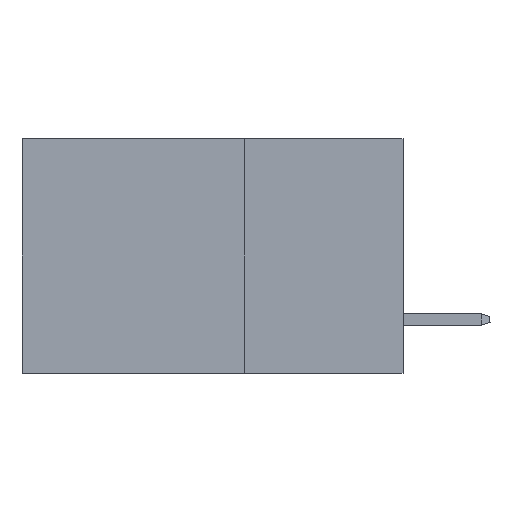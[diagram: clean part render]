
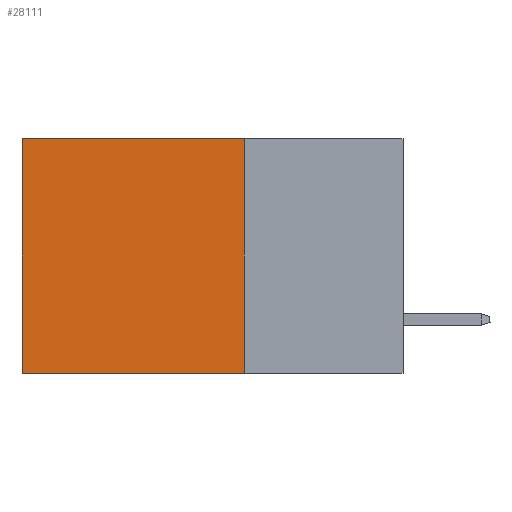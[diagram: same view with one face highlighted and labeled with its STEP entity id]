
A CAD part, left-side view. The second image highlights one B-rep face of the part: STEP entity #28111.
In plain terms, the highlighted planar face has unit normal (-1, 0, 0).
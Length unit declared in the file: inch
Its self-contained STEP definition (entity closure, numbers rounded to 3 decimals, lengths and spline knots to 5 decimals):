
#2218 = VERTEX_POINT ( 'NONE', #21784 ) ;
#2879 = ORIENTED_EDGE ( 'NONE', *, *, #13829, .T. ) ;
#3216 = FACE_OUTER_BOUND ( 'NONE', #24705, .T. ) ;
#4052 = LINE ( 'NONE', #24756, #30593 ) ;
#4526 = CARTESIAN_POINT ( 'NONE',  ( 0.2875, 0.25, 0. ) ) ;
#4668 = ORIENTED_EDGE ( 'NONE', *, *, #8769, .T. ) ;
#4880 = ORIENTED_EDGE ( 'NONE', *, *, #26706, .F. ) ;
#5278 = AXIS2_PLACEMENT_3D ( 'NONE', #7949, #16100, #31697 ) ;
#6870 = LINE ( 'NONE', #4526, #12375 ) ;
#7220 = DIRECTION ( 'NONE',  ( 0., 0., -1. ) ) ;
#7663 = VECTOR ( 'NONE', #10708, 39.37008 ) ;
#7949 = CARTESIAN_POINT ( 'NONE',  ( 0.2875, 0.25, 0. ) ) ;
#8684 = DIRECTION ( 'NONE',  ( 0., 1., 0. ) ) ;
#8769 = EDGE_CURVE ( 'NONE', #17096, #2218, #4052, .T. ) ;
#10707 = VECTOR ( 'NONE', #8684, 39.37008 ) ;
#10708 = DIRECTION ( 'NONE',  ( 0., 0., -1. ) ) ;
#11567 = CARTESIAN_POINT ( 'NONE',  ( 0.2875, 0.25, -0.37 ) ) ;
#12368 = ORIENTED_EDGE ( 'NONE', *, *, #24661, .F. ) ;
#12375 = VECTOR ( 'NONE', #7220, 39.37008 ) ;
#13093 = CARTESIAN_POINT ( 'NONE',  ( 0.2875, 0.6, 0. ) ) ;
#13829 = EDGE_CURVE ( 'NONE', #2218, #28823, #28545, .T. ) ;
#16100 = DIRECTION ( 'NONE',  ( 1., 0., 0. ) ) ;
#17096 = VERTEX_POINT ( 'NONE', #23700 ) ;
#21349 = PLANE ( 'NONE',  #5278 ) ;
#21784 = CARTESIAN_POINT ( 'NONE',  ( 0.2875, 0.6, 0. ) ) ;
#23700 = CARTESIAN_POINT ( 'NONE',  ( 0.2875, 0.25, 0. ) ) ;
#24196 = CARTESIAN_POINT ( 'NONE',  ( 0.2875, 0.25, -0.37 ) ) ;
#24661 = EDGE_CURVE ( 'NONE', #17096, #28641, #6870, .T. ) ;
#24705 = EDGE_LOOP ( 'NONE', ( #2879, #4880, #12368, #4668 ) ) ;
#24756 = CARTESIAN_POINT ( 'NONE',  ( 0.2875, 0.25, 0. ) ) ;
#25566 = CARTESIAN_POINT ( 'NONE',  ( 0.2875, 0.6, -0.37 ) ) ;
#26706 = EDGE_CURVE ( 'NONE', #28641, #28823, #29725, .T. ) ;
#27785 = DIRECTION ( 'NONE',  ( 0., 1., 0. ) ) ;
#28111 = ADVANCED_FACE ( 'NONE', ( #3216 ), #21349, .F. ) ;
#28545 = LINE ( 'NONE', #13093, #7663 ) ;
#28641 = VERTEX_POINT ( 'NONE', #24196 ) ;
#28823 = VERTEX_POINT ( 'NONE', #25566 ) ;
#29725 = LINE ( 'NONE', #11567, #10707 ) ;
#30593 = VECTOR ( 'NONE', #27785, 39.37008 ) ;
#31697 = DIRECTION ( 'NONE',  ( 0., 0., -1. ) ) ;
